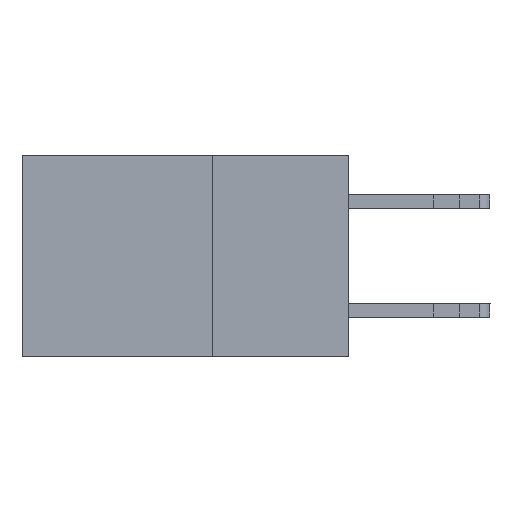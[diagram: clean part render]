
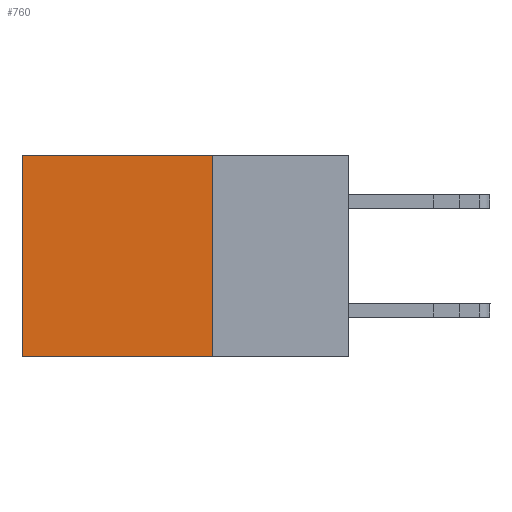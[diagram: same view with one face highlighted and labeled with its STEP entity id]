
A CAD part, left-side view. The second image highlights one B-rep face of the part: STEP entity #760.
In plain terms, the highlighted planar face has unit normal (-1, 0, 0).
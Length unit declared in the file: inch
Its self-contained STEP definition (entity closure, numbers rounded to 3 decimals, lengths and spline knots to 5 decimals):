
#396 = VERTEX_POINT ( 'NONE', #4116 ) ;
#752 = DIRECTION ( 'NONE',  ( 0., 1., 0. ) ) ;
#760 = ADVANCED_FACE ( 'NONE', ( #7617 ), #832, .F. ) ;
#832 = PLANE ( 'NONE',  #6079 ) ;
#880 = CARTESIAN_POINT ( 'NONE',  ( 0.2615, 0.6, -0.37 ) ) ;
#1266 = CARTESIAN_POINT ( 'NONE',  ( 0.2615, 0.25, -0.37 ) ) ;
#1602 = EDGE_CURVE ( 'NONE', #11062, #396, #5553, .T. ) ;
#1753 = VECTOR ( 'NONE', #752, 39.37008 ) ;
#1900 = EDGE_CURVE ( 'NONE', #5257, #396, #11624, .T. ) ;
#2261 = EDGE_LOOP ( 'NONE', ( #10509, #11724, #5221, #10739 ) ) ;
#3133 = VECTOR ( 'NONE', #9272, 39.37008 ) ;
#3168 = CARTESIAN_POINT ( 'NONE',  ( 0.2615, 0.6, 0. ) ) ;
#4116 = CARTESIAN_POINT ( 'NONE',  ( 0.2615, 0.6, -0.37 ) ) ;
#5221 = ORIENTED_EDGE ( 'NONE', *, *, #8491, .F. ) ;
#5257 = VERTEX_POINT ( 'NONE', #5616 ) ;
#5443 = CARTESIAN_POINT ( 'NONE',  ( 0.2615, 0.25, -0.37 ) ) ;
#5553 = LINE ( 'NONE', #880, #12209 ) ;
#5616 = CARTESIAN_POINT ( 'NONE',  ( 0.2615, 0.25, -0.37 ) ) ;
#6079 = AXIS2_PLACEMENT_3D ( 'NONE', #14247, #10820, #10695 ) ;
#6609 = DIRECTION ( 'NONE',  ( 0., 0., -1. ) ) ;
#6825 = LINE ( 'NONE', #5443, #12708 ) ;
#7362 = EDGE_CURVE ( 'NONE', #8268, #11062, #9772, .T. ) ;
#7617 = FACE_OUTER_BOUND ( 'NONE', #2261, .T. ) ;
#8125 = CARTESIAN_POINT ( 'NONE',  ( 0.2615, 0.25, 0. ) ) ;
#8268 = VERTEX_POINT ( 'NONE', #10899 ) ;
#8491 = EDGE_CURVE ( 'NONE', #8268, #5257, #6825, .T. ) ;
#9272 = DIRECTION ( 'NONE',  ( 0., 1., 0. ) ) ;
#9772 = LINE ( 'NONE', #8125, #3133 ) ;
#10509 = ORIENTED_EDGE ( 'NONE', *, *, #1602, .T. ) ;
#10695 = DIRECTION ( 'NONE',  ( 0., 0., -1. ) ) ;
#10739 = ORIENTED_EDGE ( 'NONE', *, *, #7362, .T. ) ;
#10820 = DIRECTION ( 'NONE',  ( 1., 0., 0. ) ) ;
#10899 = CARTESIAN_POINT ( 'NONE',  ( 0.2615, 0.25, 0. ) ) ;
#11062 = VERTEX_POINT ( 'NONE', #3168 ) ;
#11624 = LINE ( 'NONE', #1266, #1753 ) ;
#11724 = ORIENTED_EDGE ( 'NONE', *, *, #1900, .F. ) ;
#12209 = VECTOR ( 'NONE', #14442, 39.37008 ) ;
#12708 = VECTOR ( 'NONE', #6609, 39.37008 ) ;
#14247 = CARTESIAN_POINT ( 'NONE',  ( 0.2615, 0.25, -0.37 ) ) ;
#14442 = DIRECTION ( 'NONE',  ( 0., 0., -1. ) ) ;
